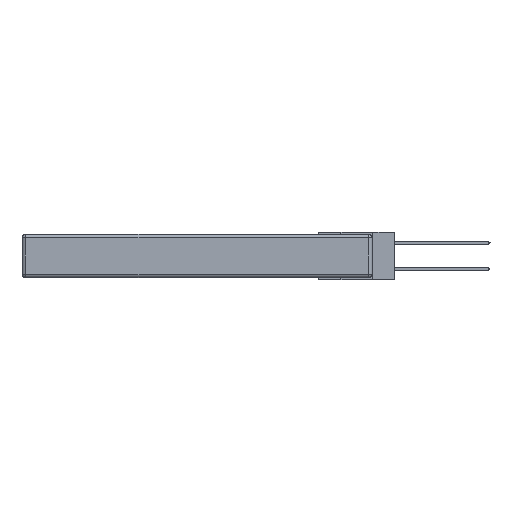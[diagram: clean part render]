
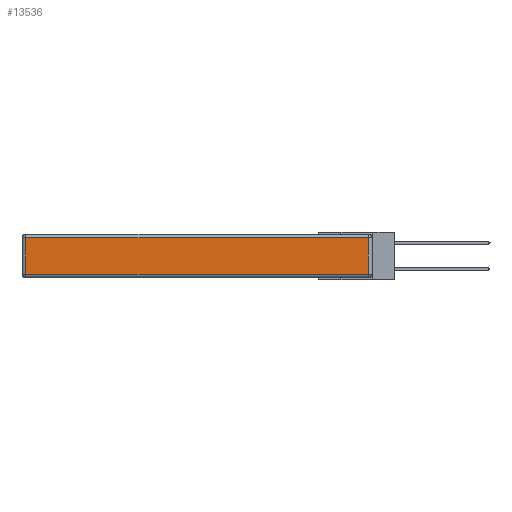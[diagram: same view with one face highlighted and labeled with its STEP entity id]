
A CAD part, left-side view. The second image highlights one B-rep face of the part: STEP entity #13536.
In plain terms, the highlighted planar face has unit normal (-1, 0, 0).
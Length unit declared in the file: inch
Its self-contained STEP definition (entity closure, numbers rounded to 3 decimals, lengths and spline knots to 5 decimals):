
#276 = VERTEX_POINT ( 'NONE', #1026 ) ;
#932 = VERTEX_POINT ( 'NONE', #12469 ) ;
#1016 = CARTESIAN_POINT ( 'NONE',  ( 0., 2.75, -0.03 ) ) ;
#1026 = CARTESIAN_POINT ( 'NONE',  ( 0., 2.72, -0.03 ) ) ;
#1728 = VERTEX_POINT ( 'NONE', #21964 ) ;
#1812 = LINE ( 'NONE', #7332, #15434 ) ;
#2367 = DIRECTION ( 'NONE',  ( 0., 0., 1. ) ) ;
#2427 = EDGE_CURVE ( 'NONE', #1728, #932, #24364, .T. ) ;
#3807 = DIRECTION ( 'NONE',  ( 0., 0., 1. ) ) ;
#6307 = LINE ( 'NONE', #22187, #10961 ) ;
#7026 = FACE_OUTER_BOUND ( 'NONE', #28121, .T. ) ;
#7332 = CARTESIAN_POINT ( 'NONE',  ( 0., 2.72, -0.343 ) ) ;
#9157 = PLANE ( 'NONE',  #33237 ) ;
#9497 = ORIENTED_EDGE ( 'NONE', *, *, #34808, .T. ) ;
#10961 = VECTOR ( 'NONE', #19804, 39.37008 ) ;
#12127 = DIRECTION ( 'NONE',  ( 0., 1., 0. ) ) ;
#12394 = ORIENTED_EDGE ( 'NONE', *, *, #23664, .T. ) ;
#12469 = CARTESIAN_POINT ( 'NONE',  ( 0., 0.03, -0.03 ) ) ;
#12756 = ORIENTED_EDGE ( 'NONE', *, *, #27535, .T. ) ;
#13536 = ADVANCED_FACE ( 'NONE', ( #7026 ), #9157, .T. ) ;
#14864 = CARTESIAN_POINT ( 'NONE',  ( 0., 0., -0.343 ) ) ;
#15434 = VECTOR ( 'NONE', #32182, 39.37008 ) ;
#16156 = ORIENTED_EDGE ( 'NONE', *, *, #2427, .T. ) ;
#17399 = DIRECTION ( 'NONE',  ( -1., 0., 0. ) ) ;
#19804 = DIRECTION ( 'NONE',  ( 0., -1., 0. ) ) ;
#20130 = VERTEX_POINT ( 'NONE', #25615 ) ;
#21964 = CARTESIAN_POINT ( 'NONE',  ( 0., 0.03, -0.313 ) ) ;
#22187 = CARTESIAN_POINT ( 'NONE',  ( 0., 0., -0.313 ) ) ;
#23564 = LINE ( 'NONE', #1016, #24409 ) ;
#23664 = EDGE_CURVE ( 'NONE', #276, #20130, #1812, .T. ) ;
#24364 = LINE ( 'NONE', #32463, #28656 ) ;
#24409 = VECTOR ( 'NONE', #12127, 39.37008 ) ;
#25615 = CARTESIAN_POINT ( 'NONE',  ( 0., 2.72, -0.313 ) ) ;
#27535 = EDGE_CURVE ( 'NONE', #932, #276, #23564, .T. ) ;
#28121 = EDGE_LOOP ( 'NONE', ( #9497, #16156, #12756, #12394 ) ) ;
#28656 = VECTOR ( 'NONE', #2367, 39.37008 ) ;
#32182 = DIRECTION ( 'NONE',  ( 0., 0., -1. ) ) ;
#32463 = CARTESIAN_POINT ( 'NONE',  ( 0., 0.03, -0.343 ) ) ;
#33237 = AXIS2_PLACEMENT_3D ( 'NONE', #14864, #17399, #3807 ) ;
#34808 = EDGE_CURVE ( 'NONE', #20130, #1728, #6307, .T. ) ;
